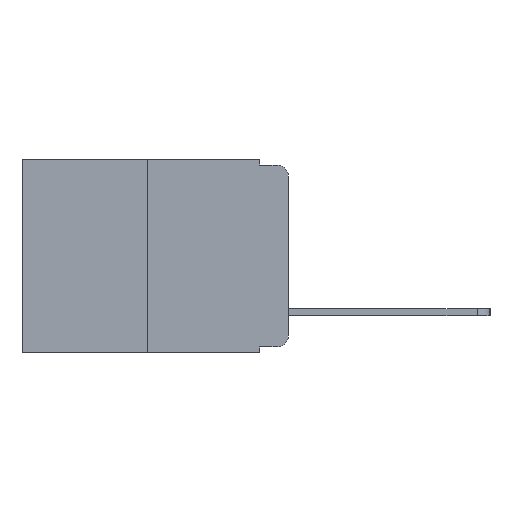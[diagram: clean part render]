
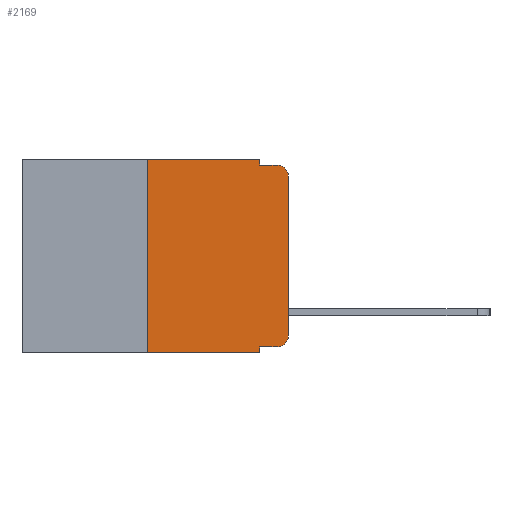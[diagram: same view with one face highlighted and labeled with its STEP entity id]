
A CAD part, left-side view. The second image highlights one B-rep face of the part: STEP entity #2169.
In plain terms, the highlighted planar face has unit normal (-1, 0, 0).
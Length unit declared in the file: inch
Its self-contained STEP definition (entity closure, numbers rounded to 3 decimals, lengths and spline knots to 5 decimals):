
#204 = DIRECTION ( 'NONE',  ( 0., 0., -1. ) ) ;
#271 = VERTEX_POINT ( 'NONE', #11496 ) ;
#594 = VERTEX_POINT ( 'NONE', #7624 ) ;
#883 = ORIENTED_EDGE ( 'NONE', *, *, #3924, .F. ) ;
#897 = CARTESIAN_POINT ( 'NONE',  ( 0., 0.051, -0.333 ) ) ;
#1472 = CARTESIAN_POINT ( 'NONE',  ( 0., 0.25, 0. ) ) ;
#2169 = ADVANCED_FACE ( 'NONE', ( #2479 ), #15231, .F. ) ;
#2372 = ORIENTED_EDGE ( 'NONE', *, *, #5976, .T. ) ;
#2479 = FACE_OUTER_BOUND ( 'NONE', #13469, .T. ) ;
#2534 = VERTEX_POINT ( 'NONE', #4866 ) ;
#2681 = VECTOR ( 'NONE', #204, 39.37008 ) ;
#2682 = VERTEX_POINT ( 'NONE', #8701 ) ;
#3116 = VECTOR ( 'NONE', #13071, 39.37008 ) ;
#3768 = DIRECTION ( 'NONE',  ( 0., -1., 0. ) ) ;
#3771 = CARTESIAN_POINT ( 'NONE',  ( 0., 0.051, -0.01 ) ) ;
#3924 = EDGE_CURVE ( 'NONE', #3959, #594, #17325, .T. ) ;
#3945 = DIRECTION ( 'NONE',  ( -1., 0., 0. ) ) ;
#3959 = VERTEX_POINT ( 'NONE', #13300 ) ;
#4038 = ORIENTED_EDGE ( 'NONE', *, *, #7330, .F. ) ;
#4060 = CARTESIAN_POINT ( 'NONE',  ( 0., 0.473, -0.343 ) ) ;
#4402 = EDGE_CURVE ( 'NONE', #2534, #12394, #12194, .T. ) ;
#4747 = CARTESIAN_POINT ( 'NONE',  ( 0., 0.051, 0. ) ) ;
#4866 = CARTESIAN_POINT ( 'NONE',  ( 0., 0.051, -0.01 ) ) ;
#5084 = CARTESIAN_POINT ( 'NONE',  ( 0., 0.051, 0. ) ) ;
#5293 = CARTESIAN_POINT ( 'NONE',  ( 0., 0.473, 0. ) ) ;
#5392 = ORIENTED_EDGE ( 'NONE', *, *, #11054, .F. ) ;
#5730 = AXIS2_PLACEMENT_3D ( 'NONE', #16297, #8287, #17612 ) ;
#5976 = EDGE_CURVE ( 'NONE', #12349, #2682, #14187, .T. ) ;
#6048 = LINE ( 'NONE', #1472, #8963 ) ;
#6550 = DIRECTION ( 'NONE',  ( 0., 0., -1. ) ) ;
#6608 = LINE ( 'NONE', #4747, #2681 ) ;
#6955 = VECTOR ( 'NONE', #12425, 39.37008 ) ;
#7216 = CIRCLE ( 'NONE', #8608, 0.02 ) ;
#7330 = EDGE_CURVE ( 'NONE', #594, #2534, #13502, .T. ) ;
#7333 = CARTESIAN_POINT ( 'NONE',  ( 0., 0.473, 0. ) ) ;
#7624 = CARTESIAN_POINT ( 'NONE',  ( 0., 0.051, 0. ) ) ;
#8059 = VERTEX_POINT ( 'NONE', #15468 ) ;
#8287 = DIRECTION ( 'NONE',  ( -1., 0., 0. ) ) ;
#8608 = AXIS2_PLACEMENT_3D ( 'NONE', #12335, #3945, #13659 ) ;
#8701 = CARTESIAN_POINT ( 'NONE',  ( 0., 0.02, -0.333 ) ) ;
#8815 = CIRCLE ( 'NONE', #5730, 0.02 ) ;
#8963 = VECTOR ( 'NONE', #10229, 39.37008 ) ;
#9590 = VECTOR ( 'NONE', #12441, 39.37008 ) ;
#9911 = CARTESIAN_POINT ( 'NONE',  ( 0., 0.051, -0.333 ) ) ;
#10229 = DIRECTION ( 'NONE',  ( 0., 0., 1. ) ) ;
#10711 = ORIENTED_EDGE ( 'NONE', *, *, #12278, .T. ) ;
#10718 = EDGE_CURVE ( 'NONE', #2682, #271, #7216, .T. ) ;
#10796 = EDGE_CURVE ( 'NONE', #18061, #17847, #17094, .T. ) ;
#11054 = EDGE_CURVE ( 'NONE', #18061, #3959, #6048, .T. ) ;
#11313 = CARTESIAN_POINT ( 'NONE',  ( 0., 0.02, -0.01 ) ) ;
#11496 = CARTESIAN_POINT ( 'NONE',  ( 0., 0., -0.313 ) ) ;
#12194 = LINE ( 'NONE', #3771, #15690 ) ;
#12278 = EDGE_CURVE ( 'NONE', #271, #8059, #13136, .T. ) ;
#12335 = CARTESIAN_POINT ( 'NONE',  ( 0., 0.02, -0.313 ) ) ;
#12349 = VERTEX_POINT ( 'NONE', #9911 ) ;
#12394 = VERTEX_POINT ( 'NONE', #11313 ) ;
#12425 = DIRECTION ( 'NONE',  ( 0., -1., 0. ) ) ;
#12441 = DIRECTION ( 'NONE',  ( 0., 0., 1. ) ) ;
#12461 = AXIS2_PLACEMENT_3D ( 'NONE', #7333, #16350, #15599 ) ;
#12776 = ORIENTED_EDGE ( 'NONE', *, *, #10796, .T. ) ;
#13071 = DIRECTION ( 'NONE',  ( 0., -1., 0. ) ) ;
#13136 = LINE ( 'NONE', #17646, #9590 ) ;
#13185 = VECTOR ( 'NONE', #13772, 39.37008 ) ;
#13300 = CARTESIAN_POINT ( 'NONE',  ( 0., 0.25, 0. ) ) ;
#13469 = EDGE_LOOP ( 'NONE', ( #10711, #17700, #14642, #4038, #883, #5392, #12776, #16695, #2372, #17514 ) ) ;
#13502 = LINE ( 'NONE', #5084, #14744 ) ;
#13659 = DIRECTION ( 'NONE',  ( 0., 0., -1. ) ) ;
#13772 = DIRECTION ( 'NONE',  ( 0., -1., 0. ) ) ;
#14187 = LINE ( 'NONE', #897, #6955 ) ;
#14642 = ORIENTED_EDGE ( 'NONE', *, *, #4402, .F. ) ;
#14744 = VECTOR ( 'NONE', #6550, 39.37008 ) ;
#15231 = PLANE ( 'NONE',  #12461 ) ;
#15453 = EDGE_CURVE ( 'NONE', #12349, #17847, #6608, .T. ) ;
#15468 = CARTESIAN_POINT ( 'NONE',  ( 0., 0., -0.03 ) ) ;
#15599 = DIRECTION ( 'NONE',  ( 0., 0., -1. ) ) ;
#15690 = VECTOR ( 'NONE', #3768, 39.37008 ) ;
#15802 = EDGE_CURVE ( 'NONE', #8059, #12394, #8815, .T. ) ;
#15875 = CARTESIAN_POINT ( 'NONE',  ( 0., 0.051, -0.343 ) ) ;
#16297 = CARTESIAN_POINT ( 'NONE',  ( 0., 0.02, -0.03 ) ) ;
#16350 = DIRECTION ( 'NONE',  ( 1., 0., 0. ) ) ;
#16695 = ORIENTED_EDGE ( 'NONE', *, *, #15453, .F. ) ;
#17094 = LINE ( 'NONE', #4060, #13185 ) ;
#17325 = LINE ( 'NONE', #5293, #3116 ) ;
#17514 = ORIENTED_EDGE ( 'NONE', *, *, #10718, .T. ) ;
#17526 = CARTESIAN_POINT ( 'NONE',  ( 0., 0.25, -0.343 ) ) ;
#17612 = DIRECTION ( 'NONE',  ( 0., 0., -1. ) ) ;
#17646 = CARTESIAN_POINT ( 'NONE',  ( 0., 0., 0. ) ) ;
#17700 = ORIENTED_EDGE ( 'NONE', *, *, #15802, .T. ) ;
#17847 = VERTEX_POINT ( 'NONE', #15875 ) ;
#18061 = VERTEX_POINT ( 'NONE', #17526 ) ;
